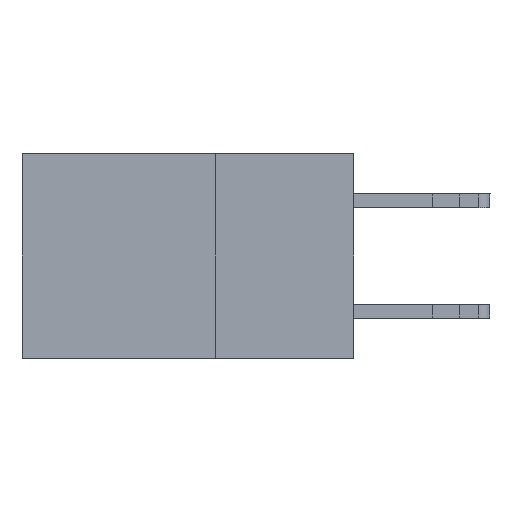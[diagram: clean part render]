
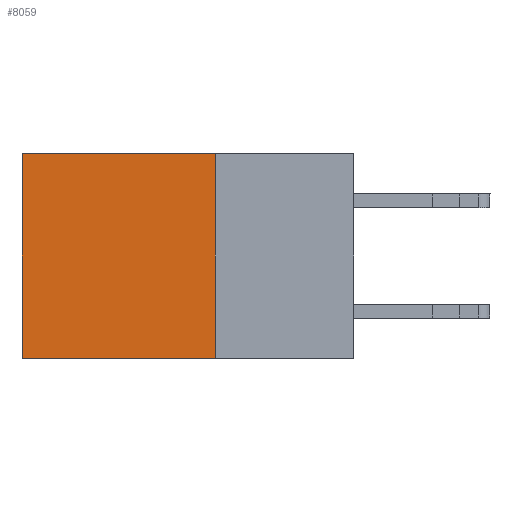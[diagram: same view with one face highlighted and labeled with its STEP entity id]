
A CAD part, left-side view. The second image highlights one B-rep face of the part: STEP entity #8059.
In plain terms, the highlighted planar face has unit normal (-1, 0, 0).
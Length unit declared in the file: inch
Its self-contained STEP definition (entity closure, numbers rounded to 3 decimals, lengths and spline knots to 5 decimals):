
#453 = ORIENTED_EDGE ( 'NONE', *, *, #11199, .T. ) ;
#1546 = DIRECTION ( 'NONE',  ( 0., 0., -1. ) ) ;
#1652 = ORIENTED_EDGE ( 'NONE', *, *, #6704, .F. ) ;
#2765 = CARTESIAN_POINT ( 'NONE',  ( 0.2875, 0.25, -0.37 ) ) ;
#3126 = LINE ( 'NONE', #5863, #10615 ) ;
#4864 = CARTESIAN_POINT ( 'NONE',  ( 0.2875, 0.6, 0. ) ) ;
#4969 = CARTESIAN_POINT ( 'NONE',  ( 0.2875, 0.25, 0. ) ) ;
#5863 = CARTESIAN_POINT ( 'NONE',  ( 0.2875, 0.25, 0. ) ) ;
#6704 = EDGE_CURVE ( 'NONE', #12544, #10770, #10025, .T. ) ;
#7822 = DIRECTION ( 'NONE',  ( 1., 0., 0. ) ) ;
#8059 = ADVANCED_FACE ( 'NONE', ( #9430 ), #9285, .F. ) ;
#8922 = EDGE_CURVE ( 'NONE', #10770, #9867, #22663, .T. ) ;
#9285 = PLANE ( 'NONE',  #13531 ) ;
#9430 = FACE_OUTER_BOUND ( 'NONE', #11677, .T. ) ;
#9867 = VERTEX_POINT ( 'NONE', #13340 ) ;
#10025 = LINE ( 'NONE', #4969, #14046 ) ;
#10615 = VECTOR ( 'NONE', #13231, 39.37008 ) ;
#10638 = CARTESIAN_POINT ( 'NONE',  ( 0.2875, 0.25, 0. ) ) ;
#10770 = VERTEX_POINT ( 'NONE', #16985 ) ;
#11199 = EDGE_CURVE ( 'NONE', #12544, #23616, #3126, .T. ) ;
#11294 = CARTESIAN_POINT ( 'NONE',  ( 0.2875, 0.25, 0. ) ) ;
#11525 = DIRECTION ( 'NONE',  ( 0., 0., -1. ) ) ;
#11677 = EDGE_LOOP ( 'NONE', ( #20880, #12203, #1652, #453 ) ) ;
#12170 = DIRECTION ( 'NONE',  ( 0., 0., -1. ) ) ;
#12203 = ORIENTED_EDGE ( 'NONE', *, *, #8922, .F. ) ;
#12544 = VERTEX_POINT ( 'NONE', #10638 ) ;
#13231 = DIRECTION ( 'NONE',  ( 0., 1., 0. ) ) ;
#13250 = VECTOR ( 'NONE', #22561, 39.37008 ) ;
#13340 = CARTESIAN_POINT ( 'NONE',  ( 0.2875, 0.6, -0.37 ) ) ;
#13531 = AXIS2_PLACEMENT_3D ( 'NONE', #11294, #7822, #11525 ) ;
#14046 = VECTOR ( 'NONE', #1546, 39.37008 ) ;
#14418 = EDGE_CURVE ( 'NONE', #23616, #9867, #15290, .T. ) ;
#15290 = LINE ( 'NONE', #4864, #22419 ) ;
#15720 = CARTESIAN_POINT ( 'NONE',  ( 0.2875, 0.6, 0. ) ) ;
#16985 = CARTESIAN_POINT ( 'NONE',  ( 0.2875, 0.25, -0.37 ) ) ;
#20880 = ORIENTED_EDGE ( 'NONE', *, *, #14418, .T. ) ;
#22419 = VECTOR ( 'NONE', #12170, 39.37008 ) ;
#22561 = DIRECTION ( 'NONE',  ( 0., 1., 0. ) ) ;
#22663 = LINE ( 'NONE', #2765, #13250 ) ;
#23616 = VERTEX_POINT ( 'NONE', #15720 ) ;
